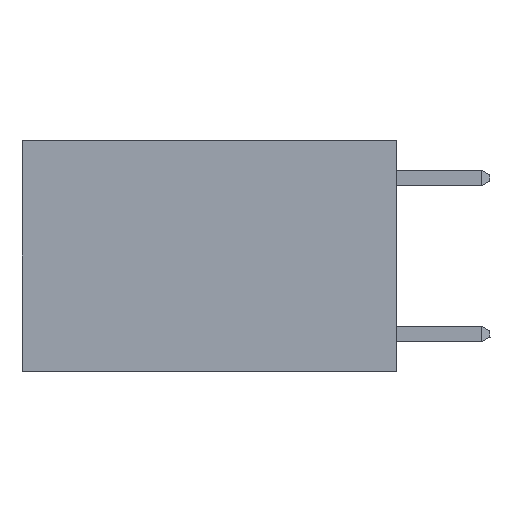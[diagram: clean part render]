
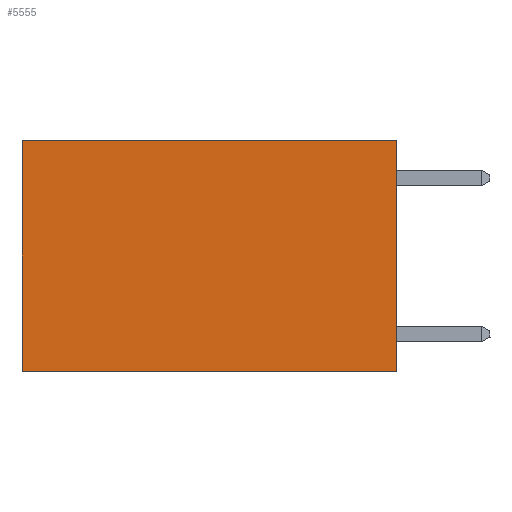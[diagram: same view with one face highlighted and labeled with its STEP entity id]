
A CAD part, left-side view. The second image highlights one B-rep face of the part: STEP entity #5555.
In plain terms, the highlighted planar face has unit normal (-1, 0, 0).
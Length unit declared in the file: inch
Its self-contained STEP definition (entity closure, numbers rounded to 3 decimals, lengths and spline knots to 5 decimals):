
#66 = EDGE_LOOP ( 'NONE', ( #8207, #8855, #8883, #12327 ) ) ;
#543 = CARTESIAN_POINT ( 'NONE',  ( 0.2625, 0., -0.37 ) ) ;
#1028 = VECTOR ( 'NONE', #13568, 39.37008 ) ;
#1099 = VERTEX_POINT ( 'NONE', #543 ) ;
#1742 = VECTOR ( 'NONE', #4632, 39.37008 ) ;
#1843 = DIRECTION ( 'NONE',  ( 0., 0., -1. ) ) ;
#1914 = CARTESIAN_POINT ( 'NONE',  ( 0.2625, 0., 0. ) ) ;
#2016 = EDGE_CURVE ( 'NONE', #1099, #12351, #4860, .T. ) ;
#2179 = EDGE_CURVE ( 'NONE', #12477, #1099, #10763, .T. ) ;
#2374 = CARTESIAN_POINT ( 'NONE',  ( 0.2625, 0., 0. ) ) ;
#3864 = EDGE_CURVE ( 'NONE', #12477, #12674, #12844, .T. ) ;
#4149 = LINE ( 'NONE', #8388, #1028 ) ;
#4273 = CARTESIAN_POINT ( 'NONE',  ( 0.2625, 0., 0. ) ) ;
#4632 = DIRECTION ( 'NONE',  ( 0., 1., 0. ) ) ;
#4781 = CARTESIAN_POINT ( 'NONE',  ( 0.2625, 0., -0.37 ) ) ;
#4860 = LINE ( 'NONE', #4781, #1742 ) ;
#5292 = DIRECTION ( 'NONE',  ( 0., 1., 0. ) ) ;
#5400 = CARTESIAN_POINT ( 'NONE',  ( 0.2625, 0., 0. ) ) ;
#5555 = ADVANCED_FACE ( 'NONE', ( #12471 ), #7684, .F. ) ;
#5708 = AXIS2_PLACEMENT_3D ( 'NONE', #5400, #12852, #6569 ) ;
#6569 = DIRECTION ( 'NONE',  ( 0., 0., -1. ) ) ;
#7367 = EDGE_CURVE ( 'NONE', #12674, #12351, #4149, .T. ) ;
#7684 = PLANE ( 'NONE',  #5708 ) ;
#8083 = VECTOR ( 'NONE', #1843, 39.37008 ) ;
#8207 = ORIENTED_EDGE ( 'NONE', *, *, #7367, .T. ) ;
#8388 = CARTESIAN_POINT ( 'NONE',  ( 0.2625, 0.6, 0. ) ) ;
#8855 = ORIENTED_EDGE ( 'NONE', *, *, #2016, .F. ) ;
#8883 = ORIENTED_EDGE ( 'NONE', *, *, #2179, .F. ) ;
#10103 = VECTOR ( 'NONE', #5292, 39.37008 ) ;
#10763 = LINE ( 'NONE', #2374, #8083 ) ;
#11751 = CARTESIAN_POINT ( 'NONE',  ( 0.2625, 0.6, 0. ) ) ;
#12327 = ORIENTED_EDGE ( 'NONE', *, *, #3864, .T. ) ;
#12351 = VERTEX_POINT ( 'NONE', #12436 ) ;
#12436 = CARTESIAN_POINT ( 'NONE',  ( 0.2625, 0.6, -0.37 ) ) ;
#12471 = FACE_OUTER_BOUND ( 'NONE', #66, .T. ) ;
#12477 = VERTEX_POINT ( 'NONE', #1914 ) ;
#12674 = VERTEX_POINT ( 'NONE', #11751 ) ;
#12844 = LINE ( 'NONE', #4273, #10103 ) ;
#12852 = DIRECTION ( 'NONE',  ( 1., 0., 0. ) ) ;
#13568 = DIRECTION ( 'NONE',  ( 0., 0., -1. ) ) ;
